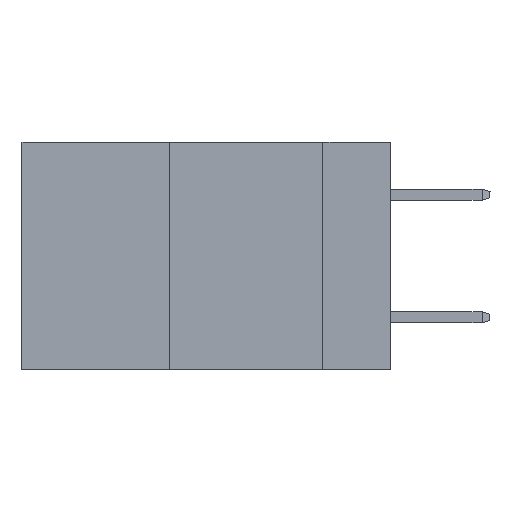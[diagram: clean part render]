
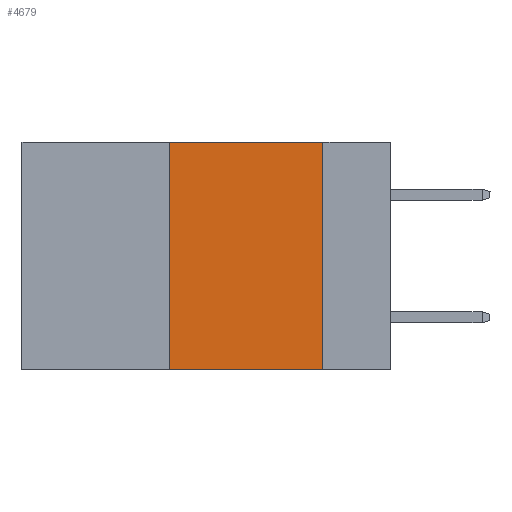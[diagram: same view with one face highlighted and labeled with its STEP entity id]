
A CAD part, left-side view. The second image highlights one B-rep face of the part: STEP entity #4679.
In plain terms, the highlighted planar face has unit normal (-1, 0, 0).
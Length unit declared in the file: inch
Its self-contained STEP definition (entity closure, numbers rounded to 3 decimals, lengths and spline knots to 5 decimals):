
#281 = VECTOR ( 'NONE', #11859, 39.37008 ) ;
#867 = LINE ( 'NONE', #22619, #281 ) ;
#890 = DIRECTION ( 'NONE',  ( 0., -1., 0. ) ) ;
#1113 = VERTEX_POINT ( 'NONE', #16681 ) ;
#2121 = CARTESIAN_POINT ( 'NONE',  ( 0., 0.11, -0.37 ) ) ;
#2146 = CARTESIAN_POINT ( 'NONE',  ( 0., 0.6, 0. ) ) ;
#2361 = PLANE ( 'NONE',  #15129 ) ;
#2787 = VERTEX_POINT ( 'NONE', #8005 ) ;
#2820 = CARTESIAN_POINT ( 'NONE',  ( 0., 0.6, -0.37 ) ) ;
#3424 = VECTOR ( 'NONE', #890, 39.37008 ) ;
#4679 = ADVANCED_FACE ( 'NONE', ( #20385 ), #2361, .F. ) ;
#7398 = ORIENTED_EDGE ( 'NONE', *, *, #19419, .F. ) ;
#8005 = CARTESIAN_POINT ( 'NONE',  ( 0., 0.36, -0.37 ) ) ;
#9088 = ORIENTED_EDGE ( 'NONE', *, *, #10976, .T. ) ;
#9413 = EDGE_CURVE ( 'NONE', #1113, #14518, #18477, .T. ) ;
#9907 = DIRECTION ( 'NONE',  ( 0., 0., -1. ) ) ;
#10976 = EDGE_CURVE ( 'NONE', #2787, #12846, #18066, .T. ) ;
#11859 = DIRECTION ( 'NONE',  ( 0., 0., -1. ) ) ;
#12084 = VECTOR ( 'NONE', #16724, 39.37008 ) ;
#12846 = VERTEX_POINT ( 'NONE', #2121 ) ;
#13127 = VECTOR ( 'NONE', #20456, 39.37008 ) ;
#13462 = CARTESIAN_POINT ( 'NONE',  ( 0., 0.6, 0. ) ) ;
#13837 = EDGE_LOOP ( 'NONE', ( #22937, #21231, #7398, #9088 ) ) ;
#14138 = EDGE_CURVE ( 'NONE', #14518, #12846, #867, .T. ) ;
#14518 = VERTEX_POINT ( 'NONE', #18986 ) ;
#15129 = AXIS2_PLACEMENT_3D ( 'NONE', #13462, #20745, #9907 ) ;
#16298 = LINE ( 'NONE', #18528, #12084 ) ;
#16681 = CARTESIAN_POINT ( 'NONE',  ( 0., 0.36, 0. ) ) ;
#16724 = DIRECTION ( 'NONE',  ( 0., 0., 1. ) ) ;
#18066 = LINE ( 'NONE', #2820, #3424 ) ;
#18477 = LINE ( 'NONE', #2146, #13127 ) ;
#18528 = CARTESIAN_POINT ( 'NONE',  ( 0., 0.36, 0. ) ) ;
#18986 = CARTESIAN_POINT ( 'NONE',  ( 0., 0.11, 0. ) ) ;
#19419 = EDGE_CURVE ( 'NONE', #2787, #1113, #16298, .T. ) ;
#20385 = FACE_OUTER_BOUND ( 'NONE', #13837, .T. ) ;
#20456 = DIRECTION ( 'NONE',  ( 0., -1., 0. ) ) ;
#20745 = DIRECTION ( 'NONE',  ( 1., 0., 0. ) ) ;
#21231 = ORIENTED_EDGE ( 'NONE', *, *, #9413, .F. ) ;
#22619 = CARTESIAN_POINT ( 'NONE',  ( 0., 0.11, 0. ) ) ;
#22937 = ORIENTED_EDGE ( 'NONE', *, *, #14138, .F. ) ;
